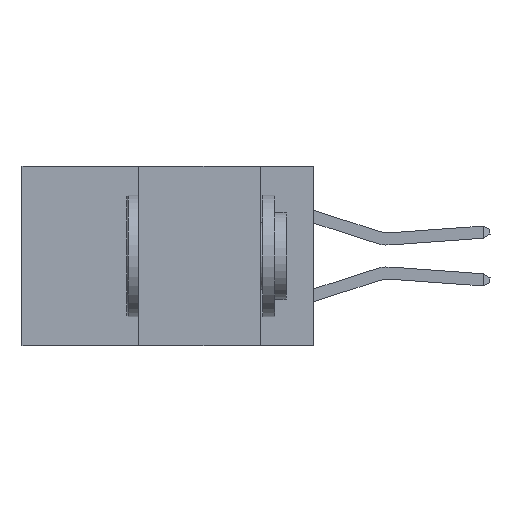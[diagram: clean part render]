
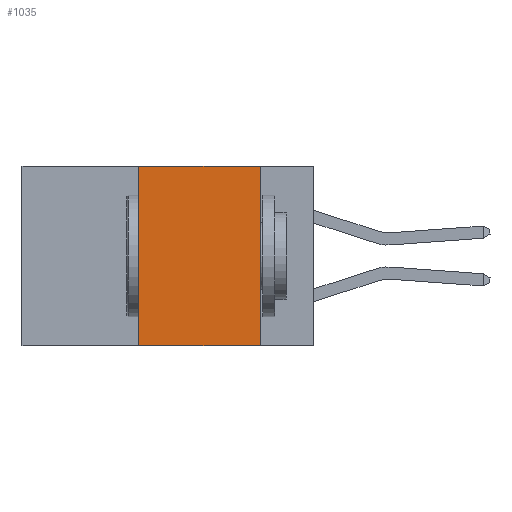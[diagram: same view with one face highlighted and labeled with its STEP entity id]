
A CAD part, left-side view. The second image highlights one B-rep face of the part: STEP entity #1035.
In plain terms, the highlighted planar face has unit normal (-1, 0, 0).
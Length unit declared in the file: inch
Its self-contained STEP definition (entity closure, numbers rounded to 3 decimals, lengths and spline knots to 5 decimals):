
#550 = VECTOR ( 'NONE', #7537, 39.37008 ) ;
#961 = DIRECTION ( 'NONE',  ( 0., -1., 0. ) ) ;
#1035 = ADVANCED_FACE ( 'NONE', ( #11057 ), #3755, .F. ) ;
#1142 = LINE ( 'NONE', #5465, #4392 ) ;
#1672 = EDGE_CURVE ( 'NONE', #5720, #4727, #10312, .T. ) ;
#1841 = DIRECTION ( 'NONE',  ( 0., 0., -1. ) ) ;
#2093 = CARTESIAN_POINT ( 'NONE',  ( 0., 0.36, 0. ) ) ;
#2407 = CARTESIAN_POINT ( 'NONE',  ( 0., 0.36, -0.37 ) ) ;
#3053 = ORIENTED_EDGE ( 'NONE', *, *, #7397, .F. ) ;
#3331 = DIRECTION ( 'NONE',  ( 0., -1., 0. ) ) ;
#3407 = VERTEX_POINT ( 'NONE', #5675 ) ;
#3614 = CARTESIAN_POINT ( 'NONE',  ( 0., 0.11, 0. ) ) ;
#3755 = PLANE ( 'NONE',  #10854 ) ;
#4054 = VECTOR ( 'NONE', #1841, 39.37008 ) ;
#4392 = VECTOR ( 'NONE', #961, 39.37008 ) ;
#4621 = ORIENTED_EDGE ( 'NONE', *, *, #1672, .F. ) ;
#4714 = ORIENTED_EDGE ( 'NONE', *, *, #6313, .T. ) ;
#4727 = VERTEX_POINT ( 'NONE', #5066 ) ;
#4761 = LINE ( 'NONE', #3614, #4054 ) ;
#5066 = CARTESIAN_POINT ( 'NONE',  ( 0., 0.36, 0. ) ) ;
#5465 = CARTESIAN_POINT ( 'NONE',  ( 0., 0.6, -0.37 ) ) ;
#5675 = CARTESIAN_POINT ( 'NONE',  ( 0., 0.11, 0. ) ) ;
#5720 = VERTEX_POINT ( 'NONE', #2407 ) ;
#6313 = EDGE_CURVE ( 'NONE', #5720, #7245, #1142, .T. ) ;
#6654 = EDGE_LOOP ( 'NONE', ( #9387, #3053, #4621, #4714 ) ) ;
#6704 = DIRECTION ( 'NONE',  ( 1., 0., 0. ) ) ;
#6971 = CARTESIAN_POINT ( 'NONE',  ( 0., 0.6, 0. ) ) ;
#7245 = VERTEX_POINT ( 'NONE', #10640 ) ;
#7397 = EDGE_CURVE ( 'NONE', #4727, #3407, #10194, .T. ) ;
#7537 = DIRECTION ( 'NONE',  ( 0., 0., 1. ) ) ;
#7646 = DIRECTION ( 'NONE',  ( 0., 0., -1. ) ) ;
#8330 = CARTESIAN_POINT ( 'NONE',  ( 0., 0.6, 0. ) ) ;
#9387 = ORIENTED_EDGE ( 'NONE', *, *, #11158, .F. ) ;
#9909 = VECTOR ( 'NONE', #3331, 39.37008 ) ;
#10194 = LINE ( 'NONE', #6971, #9909 ) ;
#10312 = LINE ( 'NONE', #2093, #550 ) ;
#10640 = CARTESIAN_POINT ( 'NONE',  ( 0., 0.11, -0.37 ) ) ;
#10854 = AXIS2_PLACEMENT_3D ( 'NONE', #8330, #6704, #7646 ) ;
#11057 = FACE_OUTER_BOUND ( 'NONE', #6654, .T. ) ;
#11158 = EDGE_CURVE ( 'NONE', #3407, #7245, #4761, .T. ) ;
